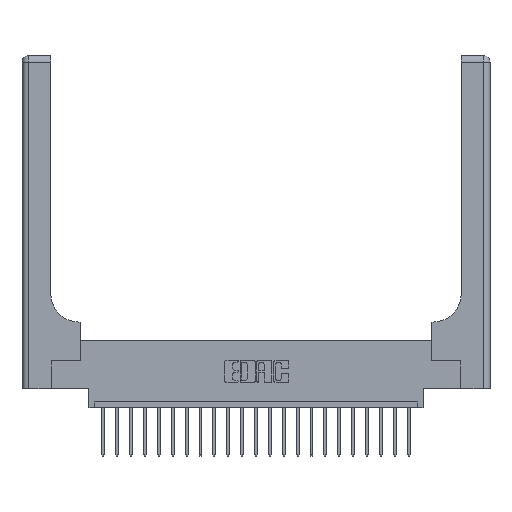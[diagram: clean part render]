
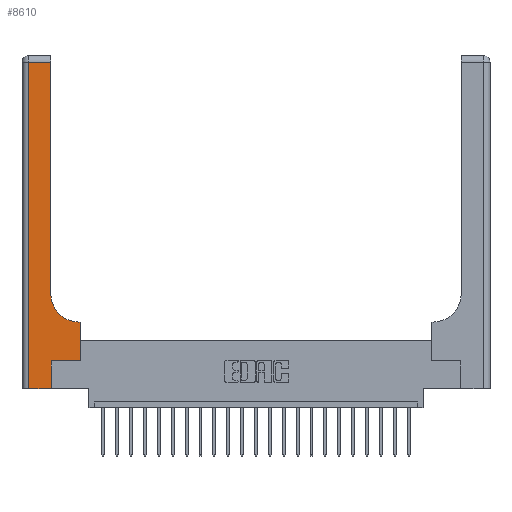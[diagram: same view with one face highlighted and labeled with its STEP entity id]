
A CAD part, top view. The second image highlights one B-rep face of the part: STEP entity #8610.
In plain terms, the highlighted planar face has unit normal (0, 0, 1).
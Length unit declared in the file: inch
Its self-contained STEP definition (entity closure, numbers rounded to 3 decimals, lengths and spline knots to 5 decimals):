
#470 = DIRECTION ( 'NONE',  ( -1., 0., 0. ) ) ;
#578 = ORIENTED_EDGE ( 'NONE', *, *, #21860, .T. ) ;
#1460 = DIRECTION ( 'NONE',  ( 1., 0., 0. ) ) ;
#1468 = EDGE_CURVE ( 'NONE', #19256, #1895, #2885, .T. ) ;
#1895 = VERTEX_POINT ( 'NONE', #10821 ) ;
#2044 = CARTESIAN_POINT ( 'NONE',  ( 0.26, 0.85, 0.37 ) ) ;
#2269 = CARTESIAN_POINT ( 'NONE',  ( 0.26, 0.6, 0.37 ) ) ;
#2885 = LINE ( 'NONE', #3190, #12540 ) ;
#2948 = CARTESIAN_POINT ( 'NONE',  ( 0.265, 0., 0.37 ) ) ;
#3190 = CARTESIAN_POINT ( 'NONE',  ( 0., 0., 0.37 ) ) ;
#3532 = ORIENTED_EDGE ( 'NONE', *, *, #18648, .T. ) ;
#4100 = LINE ( 'NONE', #9897, #20688 ) ;
#4102 = VERTEX_POINT ( 'NONE', #20787 ) ;
#4141 = ORIENTED_EDGE ( 'NONE', *, *, #10321, .T. ) ;
#4493 = EDGE_CURVE ( 'NONE', #17249, #12314, #4100, .T. ) ;
#4508 = FACE_OUTER_BOUND ( 'NONE', #10526, .T. ) ;
#5173 = ORIENTED_EDGE ( 'NONE', *, *, #17219, .T. ) ;
#7130 = DIRECTION ( 'NONE',  ( -1., 0., 0. ) ) ;
#7287 = VECTOR ( 'NONE', #7372, 39.37008 ) ;
#7372 = DIRECTION ( 'NONE',  ( 0., 1., 0. ) ) ;
#7591 = ORIENTED_EDGE ( 'NONE', *, *, #4493, .T. ) ;
#7648 = ORIENTED_EDGE ( 'NONE', *, *, #14731, .T. ) ;
#8610 = ADVANCED_FACE ( 'NONE', ( #4508 ), #16925, .F. ) ;
#8863 = CARTESIAN_POINT ( 'NONE',  ( 0.528, 0.25, 0.37 ) ) ;
#8998 = LINE ( 'NONE', #17133, #9817 ) ;
#9423 = CARTESIAN_POINT ( 'NONE',  ( 0.26, 2.94, 0.37 ) ) ;
#9817 = VECTOR ( 'NONE', #15688, 39.37008 ) ;
#9897 = CARTESIAN_POINT ( 'NONE',  ( 0.26, 3., 0.37 ) ) ;
#10174 = VECTOR ( 'NONE', #13436, 39.37008 ) ;
#10321 = EDGE_CURVE ( 'NONE', #4102, #17276, #17625, .T. ) ;
#10526 = EDGE_LOOP ( 'NONE', ( #7591, #17337, #7648, #15350, #12763, #4141, #5173, #578, #3532 ) ) ;
#10821 = CARTESIAN_POINT ( 'NONE',  ( 0.265, 0., 0.37 ) ) ;
#10916 = VECTOR ( 'NONE', #13087, 39.37008 ) ;
#11073 = AXIS2_PLACEMENT_3D ( 'NONE', #20785, #20920, #7130 ) ;
#11199 = EDGE_CURVE ( 'NONE', #12314, #11561, #12242, .T. ) ;
#11561 = VERTEX_POINT ( 'NONE', #16027 ) ;
#11825 = LINE ( 'NONE', #19149, #7287 ) ;
#12032 = CIRCLE ( 'NONE', #21306, 0.25 ) ;
#12242 = LINE ( 'NONE', #18217, #10916 ) ;
#12313 = VECTOR ( 'NONE', #470, 39.37008 ) ;
#12314 = VERTEX_POINT ( 'NONE', #9423 ) ;
#12540 = VECTOR ( 'NONE', #1460, 39.37008 ) ;
#12763 = ORIENTED_EDGE ( 'NONE', *, *, #22032, .T. ) ;
#13087 = DIRECTION ( 'NONE',  ( -1., 0., 0. ) ) ;
#13436 = DIRECTION ( 'NONE',  ( 0., 1., 0. ) ) ;
#14731 = EDGE_CURVE ( 'NONE', #11561, #19256, #8998, .T. ) ;
#15237 = DIRECTION ( 'NONE',  ( 1., 0., 0. ) ) ;
#15350 = ORIENTED_EDGE ( 'NONE', *, *, #1468, .T. ) ;
#15525 = CARTESIAN_POINT ( 'NONE',  ( 0.51, 0.6, 0.37 ) ) ;
#15688 = DIRECTION ( 'NONE',  ( 0., -1., 0. ) ) ;
#16027 = CARTESIAN_POINT ( 'NONE',  ( 0.06, 2.94, 0.37 ) ) ;
#16056 = LINE ( 'NONE', #2269, #12313 ) ;
#16598 = CARTESIAN_POINT ( 'NONE',  ( 0.06, 0., 0.37 ) ) ;
#16770 = CARTESIAN_POINT ( 'NONE',  ( 0.51, 0.85, 0.37 ) ) ;
#16925 = PLANE ( 'NONE',  #11073 ) ;
#17133 = CARTESIAN_POINT ( 'NONE',  ( 0.06, 3., 0.37 ) ) ;
#17219 = EDGE_CURVE ( 'NONE', #17276, #19565, #11825, .T. ) ;
#17249 = VERTEX_POINT ( 'NONE', #2044 ) ;
#17276 = VERTEX_POINT ( 'NONE', #8863 ) ;
#17337 = ORIENTED_EDGE ( 'NONE', *, *, #11199, .T. ) ;
#17625 = LINE ( 'NONE', #21945, #20549 ) ;
#17919 = CARTESIAN_POINT ( 'NONE',  ( 0.528, 0.6, 0.37 ) ) ;
#18217 = CARTESIAN_POINT ( 'NONE',  ( 0., 2.94, 0.37 ) ) ;
#18648 = EDGE_CURVE ( 'NONE', #19317, #17249, #12032, .T. ) ;
#19149 = CARTESIAN_POINT ( 'NONE',  ( 0.528, 0.25, 0.37 ) ) ;
#19256 = VERTEX_POINT ( 'NONE', #16598 ) ;
#19317 = VERTEX_POINT ( 'NONE', #15525 ) ;
#19565 = VERTEX_POINT ( 'NONE', #17919 ) ;
#20033 = LINE ( 'NONE', #2948, #10174 ) ;
#20166 = DIRECTION ( 'NONE',  ( 0., 1., 0. ) ) ;
#20549 = VECTOR ( 'NONE', #15237, 39.37008 ) ;
#20688 = VECTOR ( 'NONE', #20166, 39.37008 ) ;
#20785 = CARTESIAN_POINT ( 'NONE',  ( 0., 3., 0.37 ) ) ;
#20787 = CARTESIAN_POINT ( 'NONE',  ( 0.265, 0.25, 0.37 ) ) ;
#20920 = DIRECTION ( 'NONE',  ( 0., 0., -1. ) ) ;
#21306 = AXIS2_PLACEMENT_3D ( 'NONE', #16770, #21675, #21604 ) ;
#21604 = DIRECTION ( 'NONE',  ( 1., 0., 0. ) ) ;
#21675 = DIRECTION ( 'NONE',  ( 0., 0., -1. ) ) ;
#21860 = EDGE_CURVE ( 'NONE', #19565, #19317, #16056, .T. ) ;
#21945 = CARTESIAN_POINT ( 'NONE',  ( 0.265, 0.25, 0.37 ) ) ;
#22032 = EDGE_CURVE ( 'NONE', #1895, #4102, #20033, .T. ) ;
